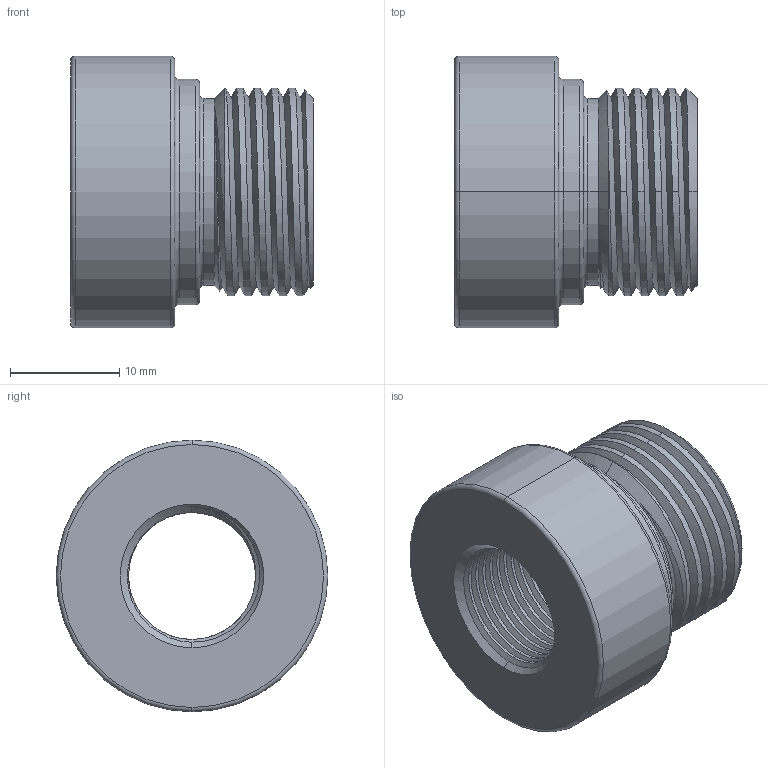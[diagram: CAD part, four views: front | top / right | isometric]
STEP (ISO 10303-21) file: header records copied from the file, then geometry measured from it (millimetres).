
FILE_DESCRIPTION (( 'STEP AP214' ), '1' );
FILE_NAME ('Adapter-P-.5-28-to-.75-16.STEP', '2013-06-18T15:14:19', ( 'Asher' ), ( '' ), 'SwSTEP 2.0', 'SolidWorks 2013', '' );
FILE_SCHEMA (( 'AUTOMOTIVE_DESIGN' ));
Length unit declared in the file: millimetre
Products named in the file (1): Adapter-P-.5-28-to-.75-16
Bounding box: 22.23 x 24.89 x 24.89 mm (x, y, z)
Volume: 5106.9 mm3; surface area: 3605.4 mm2
Topology: 1 solids, 1 shells, 70 faces, 179 edges, 113 vertices
Faces by surface type: cylinder 40, torus 12, cone 10, plane 4, bspline 4
Entity records: 4315 total; most frequent: CARTESIAN_POINT 2777, ORIENTED_EDGE 358, DIRECTION 284, EDGE_CURVE 179, AXIS2_PLACEMENT_3D 118, VERTEX_POINT 113, EDGE_LOOP 74, ADVANCED_FACE 70
